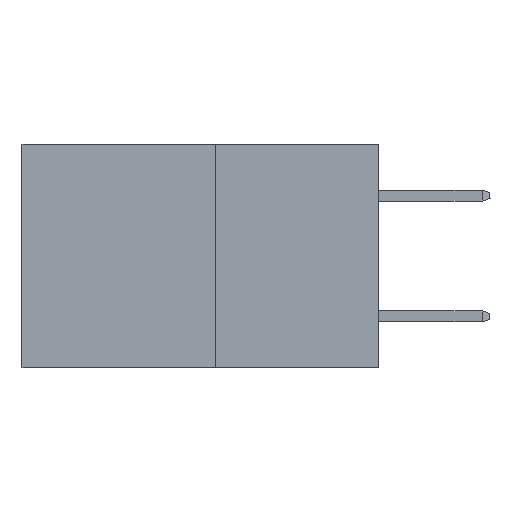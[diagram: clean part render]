
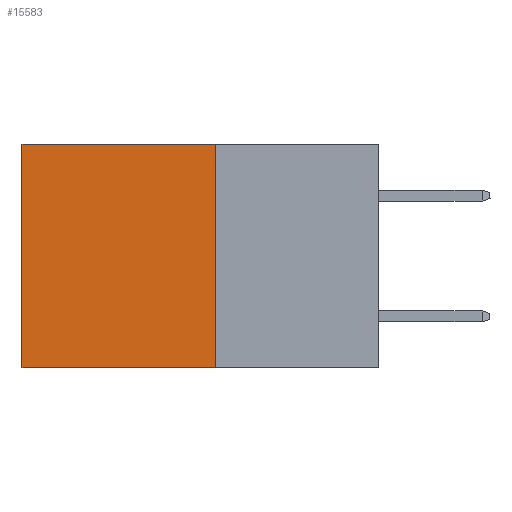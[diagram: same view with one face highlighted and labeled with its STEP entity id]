
A CAD part, left-side view. The second image highlights one B-rep face of the part: STEP entity #15583.
In plain terms, the highlighted planar face has unit normal (-1, 0, 0).
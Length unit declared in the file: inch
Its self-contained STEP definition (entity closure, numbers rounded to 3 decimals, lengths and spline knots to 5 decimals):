
#1868 = CARTESIAN_POINT ( 'NONE',  ( 0.277, 0.27, 0. ) ) ;
#2503 = CARTESIAN_POINT ( 'NONE',  ( 0.277, 0.27, -0.37 ) ) ;
#3259 = DIRECTION ( 'NONE',  ( 0., 0., -1. ) ) ;
#3413 = PLANE ( 'NONE',  #17865 ) ;
#3477 = ORIENTED_EDGE ( 'NONE', *, *, #19862, .T. ) ;
#3598 = DIRECTION ( 'NONE',  ( 0., 1., 0. ) ) ;
#4198 = CARTESIAN_POINT ( 'NONE',  ( 0.277, 0.59, 0. ) ) ;
#5750 = VECTOR ( 'NONE', #3598, 39.37008 ) ;
#5999 = DIRECTION ( 'NONE',  ( 0., 1., 0. ) ) ;
#6607 = FACE_OUTER_BOUND ( 'NONE', #7348, .T. ) ;
#6907 = DIRECTION ( 'NONE',  ( 1., 0., 0. ) ) ;
#7348 = EDGE_LOOP ( 'NONE', ( #3477, #9113, #18357, #16892 ) ) ;
#7796 = CARTESIAN_POINT ( 'NONE',  ( 0.277, 0.59, -0.37 ) ) ;
#7854 = LINE ( 'NONE', #11972, #11987 ) ;
#8143 = VECTOR ( 'NONE', #5999, 39.37008 ) ;
#8836 = VERTEX_POINT ( 'NONE', #4198 ) ;
#9113 = ORIENTED_EDGE ( 'NONE', *, *, #19162, .F. ) ;
#10160 = CARTESIAN_POINT ( 'NONE',  ( 0.277, 0.27, -0.37 ) ) ;
#10681 = EDGE_CURVE ( 'NONE', #18123, #8836, #15035, .T. ) ;
#11972 = CARTESIAN_POINT ( 'NONE',  ( 0.277, 0.27, -0.37 ) ) ;
#11987 = VECTOR ( 'NONE', #3259, 39.37008 ) ;
#12510 = LINE ( 'NONE', #7796, #16577 ) ;
#15035 = LINE ( 'NONE', #1868, #5750 ) ;
#15583 = ADVANCED_FACE ( 'NONE', ( #6607 ), #3413, .F. ) ;
#16242 = VERTEX_POINT ( 'NONE', #10160 ) ;
#16577 = VECTOR ( 'NONE', #21723, 39.37008 ) ;
#16892 = ORIENTED_EDGE ( 'NONE', *, *, #10681, .T. ) ;
#17349 = CARTESIAN_POINT ( 'NONE',  ( 0.277, 0.27, -0.37 ) ) ;
#17434 = LINE ( 'NONE', #2503, #8143 ) ;
#17668 = VERTEX_POINT ( 'NONE', #21058 ) ;
#17865 = AXIS2_PLACEMENT_3D ( 'NONE', #17349, #6907, #19108 ) ;
#18123 = VERTEX_POINT ( 'NONE', #22496 ) ;
#18357 = ORIENTED_EDGE ( 'NONE', *, *, #19418, .F. ) ;
#19108 = DIRECTION ( 'NONE',  ( 0., 0., -1. ) ) ;
#19162 = EDGE_CURVE ( 'NONE', #16242, #17668, #17434, .T. ) ;
#19418 = EDGE_CURVE ( 'NONE', #18123, #16242, #7854, .T. ) ;
#19862 = EDGE_CURVE ( 'NONE', #8836, #17668, #12510, .T. ) ;
#21058 = CARTESIAN_POINT ( 'NONE',  ( 0.277, 0.59, -0.37 ) ) ;
#21723 = DIRECTION ( 'NONE',  ( 0., 0., -1. ) ) ;
#22496 = CARTESIAN_POINT ( 'NONE',  ( 0.277, 0.27, 0. ) ) ;
